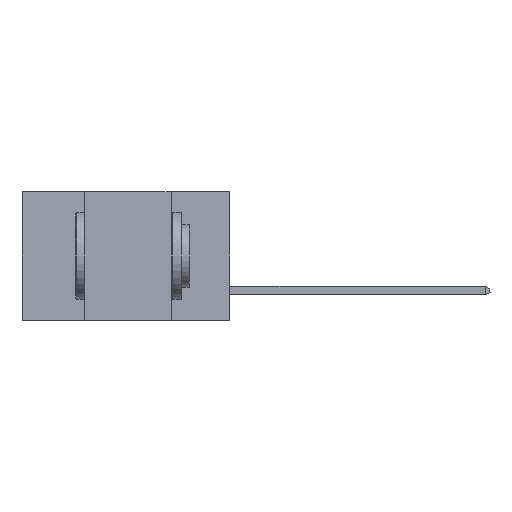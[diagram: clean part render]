
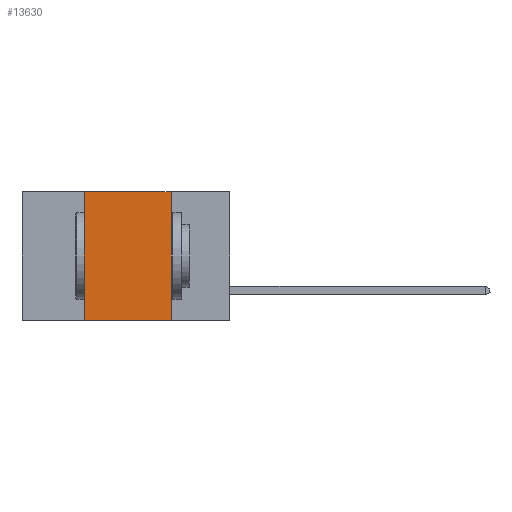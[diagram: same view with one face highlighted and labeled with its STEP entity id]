
A CAD part, left-side view. The second image highlights one B-rep face of the part: STEP entity #13630.
In plain terms, the highlighted planar face has unit normal (-1, 0, 0).
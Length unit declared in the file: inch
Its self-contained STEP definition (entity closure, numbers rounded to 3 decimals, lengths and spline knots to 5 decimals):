
#424 = VECTOR ( 'NONE', #1156, 39.37008 ) ;
#442 = DIRECTION ( 'NONE',  ( 0., 0., -1. ) ) ;
#666 = EDGE_LOOP ( 'NONE', ( #911, #16387, #8820, #3302 ) ) ;
#911 = ORIENTED_EDGE ( 'NONE', *, *, #11651, .F. ) ;
#915 = CARTESIAN_POINT ( 'NONE',  ( 0., 0.42, 0. ) ) ;
#1156 = DIRECTION ( 'NONE',  ( 0., 0., 1. ) ) ;
#1455 = CARTESIAN_POINT ( 'NONE',  ( 0., 0.17, -0.37 ) ) ;
#3025 = DIRECTION ( 'NONE',  ( 0., 0., -1. ) ) ;
#3123 = EDGE_CURVE ( 'NONE', #14828, #10779, #14568, .T. ) ;
#3302 = ORIENTED_EDGE ( 'NONE', *, *, #3841, .T. ) ;
#3841 = EDGE_CURVE ( 'NONE', #14828, #14451, #14734, .T. ) ;
#3974 = CARTESIAN_POINT ( 'NONE',  ( 0., 0.42, 0. ) ) ;
#4093 = CARTESIAN_POINT ( 'NONE',  ( 0., 0.6, 0. ) ) ;
#4499 = LINE ( 'NONE', #11454, #9550 ) ;
#4691 = VERTEX_POINT ( 'NONE', #7719 ) ;
#7719 = CARTESIAN_POINT ( 'NONE',  ( 0., 0.17, 0. ) ) ;
#7988 = CARTESIAN_POINT ( 'NONE',  ( 0., 0.42, -0.37 ) ) ;
#8820 = ORIENTED_EDGE ( 'NONE', *, *, #3123, .F. ) ;
#8866 = PLANE ( 'NONE',  #9364 ) ;
#9364 = AXIS2_PLACEMENT_3D ( 'NONE', #11586, #11531, #442 ) ;
#9550 = VECTOR ( 'NONE', #3025, 39.37008 ) ;
#10596 = FACE_OUTER_BOUND ( 'NONE', #666, .T. ) ;
#10779 = VERTEX_POINT ( 'NONE', #915 ) ;
#11068 = CARTESIAN_POINT ( 'NONE',  ( 0., 0.6, -0.37 ) ) ;
#11454 = CARTESIAN_POINT ( 'NONE',  ( 0., 0.17, 0. ) ) ;
#11531 = DIRECTION ( 'NONE',  ( 1., 0., 0. ) ) ;
#11586 = CARTESIAN_POINT ( 'NONE',  ( 0., 0.6, 0. ) ) ;
#11651 = EDGE_CURVE ( 'NONE', #4691, #14451, #4499, .T. ) ;
#12120 = VECTOR ( 'NONE', #18321, 39.37008 ) ;
#12503 = DIRECTION ( 'NONE',  ( 0., -1., 0. ) ) ;
#12581 = LINE ( 'NONE', #4093, #12120 ) ;
#13630 = ADVANCED_FACE ( 'NONE', ( #10596 ), #8866, .F. ) ;
#14451 = VERTEX_POINT ( 'NONE', #1455 ) ;
#14535 = VECTOR ( 'NONE', #12503, 39.37008 ) ;
#14568 = LINE ( 'NONE', #3974, #424 ) ;
#14734 = LINE ( 'NONE', #11068, #14535 ) ;
#14828 = VERTEX_POINT ( 'NONE', #7988 ) ;
#15331 = EDGE_CURVE ( 'NONE', #10779, #4691, #12581, .T. ) ;
#16387 = ORIENTED_EDGE ( 'NONE', *, *, #15331, .F. ) ;
#18321 = DIRECTION ( 'NONE',  ( 0., -1., 0. ) ) ;
